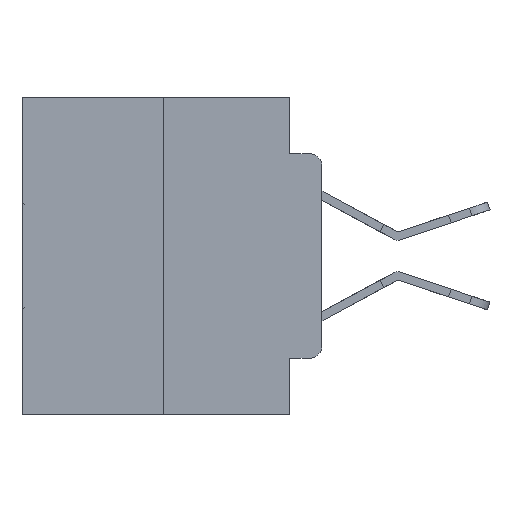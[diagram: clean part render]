
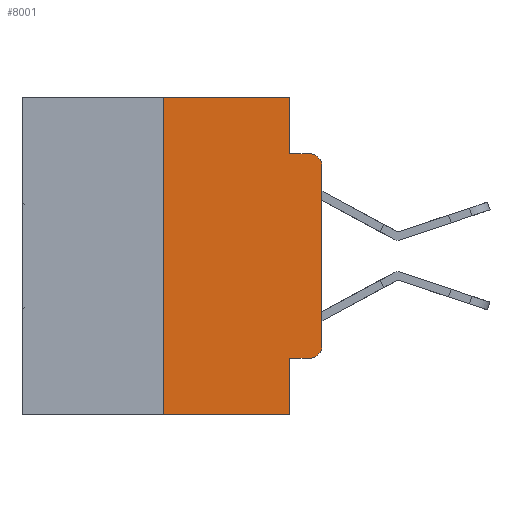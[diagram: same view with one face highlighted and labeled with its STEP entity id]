
A CAD part, left-side view. The second image highlights one B-rep face of the part: STEP entity #8001.
In plain terms, the highlighted planar face has unit normal (-1, 0, 0).
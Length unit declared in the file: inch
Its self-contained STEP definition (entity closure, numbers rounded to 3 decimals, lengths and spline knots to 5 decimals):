
#246 = VERTEX_POINT ( 'NONE', #6823 ) ;
#433 = EDGE_CURVE ( 'NONE', #11601, #15321, #3343, .T. ) ;
#1940 = CARTESIAN_POINT ( 'NONE',  ( 0., 0.02, -0.4115 ) ) ;
#2152 = LINE ( 'NONE', #27426, #26834 ) ;
#2214 = ORIENTED_EDGE ( 'NONE', *, *, #11954, .T. ) ;
#2532 = ORIENTED_EDGE ( 'NONE', *, *, #14152, .F. ) ;
#3255 = EDGE_CURVE ( 'NONE', #19969, #15321, #6133, .T. ) ;
#3343 = LINE ( 'NONE', #30752, #22006 ) ;
#3483 = EDGE_CURVE ( 'NONE', #5431, #4644, #4280, .T. ) ;
#3608 = CARTESIAN_POINT ( 'NONE',  ( 0., 0., -0.3915 ) ) ;
#3788 = CARTESIAN_POINT ( 'NONE',  ( 0., 0.02, -0.0885 ) ) ;
#4202 = EDGE_CURVE ( 'NONE', #11601, #246, #11299, .T. ) ;
#4280 = LINE ( 'NONE', #8751, #16219 ) ;
#4644 = VERTEX_POINT ( 'NONE', #3788 ) ;
#5431 = VERTEX_POINT ( 'NONE', #14275 ) ;
#5774 = PLANE ( 'NONE',  #16772 ) ;
#5930 = DIRECTION ( 'NONE',  ( -1., 0., 0. ) ) ;
#6040 = CARTESIAN_POINT ( 'NONE',  ( 0., 0.02, -0.1085 ) ) ;
#6133 = LINE ( 'NONE', #27066, #17365 ) ;
#6452 = DIRECTION ( 'NONE',  ( -1., 0., 0. ) ) ;
#6823 = CARTESIAN_POINT ( 'NONE',  ( 0., 0.25, 0. ) ) ;
#7395 = CARTESIAN_POINT ( 'NONE',  ( 0., 0.051, 0. ) ) ;
#7549 = VERTEX_POINT ( 'NONE', #16477 ) ;
#7590 = DIRECTION ( 'NONE',  ( 0., 0., -1. ) ) ;
#7930 = ORIENTED_EDGE ( 'NONE', *, *, #27833, .T. ) ;
#8001 = ADVANCED_FACE ( 'NONE', ( #8722 ), #5774, .F. ) ;
#8009 = VERTEX_POINT ( 'NONE', #3608 ) ;
#8514 = ORIENTED_EDGE ( 'NONE', *, *, #3255, .F. ) ;
#8722 = FACE_OUTER_BOUND ( 'NONE', #22912, .T. ) ;
#8751 = CARTESIAN_POINT ( 'NONE',  ( 0., 0.051, -0.0885 ) ) ;
#9223 = ORIENTED_EDGE ( 'NONE', *, *, #3483, .F. ) ;
#9271 = CARTESIAN_POINT ( 'NONE',  ( 0., 0., -0.1085 ) ) ;
#10031 = CARTESIAN_POINT ( 'NONE',  ( 0., 0.051, -0.4115 ) ) ;
#10370 = DIRECTION ( 'NONE',  ( 0., 0., 1. ) ) ;
#10513 = EDGE_CURVE ( 'NONE', #246, #7549, #16839, .T. ) ;
#11299 = LINE ( 'NONE', #25445, #20249 ) ;
#11601 = VERTEX_POINT ( 'NONE', #18677 ) ;
#11954 = EDGE_CURVE ( 'NONE', #19969, #25583, #2152, .T. ) ;
#13089 = DIRECTION ( 'NONE',  ( 1., 0., 0. ) ) ;
#13107 = VECTOR ( 'NONE', #21830, 39.37008 ) ;
#13249 = AXIS2_PLACEMENT_3D ( 'NONE', #6040, #5930, #27075 ) ;
#13459 = DIRECTION ( 'NONE',  ( 0., 0., -1. ) ) ;
#14152 = EDGE_CURVE ( 'NONE', #7549, #5431, #26168, .T. ) ;
#14275 = CARTESIAN_POINT ( 'NONE',  ( 0., 0.051, -0.0885 ) ) ;
#15321 = VERTEX_POINT ( 'NONE', #20814 ) ;
#15499 = DIRECTION ( 'NONE',  ( 0., 0., -1. ) ) ;
#15540 = DIRECTION ( 'NONE',  ( 0., -1., 0. ) ) ;
#15926 = DIRECTION ( 'NONE',  ( 0., 0., 1. ) ) ;
#16219 = VECTOR ( 'NONE', #15540, 39.37008 ) ;
#16477 = CARTESIAN_POINT ( 'NONE',  ( 0., 0.051, 0. ) ) ;
#16772 = AXIS2_PLACEMENT_3D ( 'NONE', #24996, #13089, #15499 ) ;
#16839 = LINE ( 'NONE', #21631, #13107 ) ;
#17365 = VECTOR ( 'NONE', #22522, 39.37008 ) ;
#17809 = VERTEX_POINT ( 'NONE', #9271 ) ;
#18624 = CIRCLE ( 'NONE', #20260, 0.02 ) ;
#18677 = CARTESIAN_POINT ( 'NONE',  ( 0., 0.25, -0.5 ) ) ;
#19781 = VECTOR ( 'NONE', #7590, 39.37008 ) ;
#19969 = VERTEX_POINT ( 'NONE', #10031 ) ;
#19970 = ORIENTED_EDGE ( 'NONE', *, *, #433, .T. ) ;
#20072 = DIRECTION ( 'NONE',  ( 0., -1., 0. ) ) ;
#20249 = VECTOR ( 'NONE', #15926, 39.37008 ) ;
#20260 = AXIS2_PLACEMENT_3D ( 'NONE', #23148, #6452, #13459 ) ;
#20814 = CARTESIAN_POINT ( 'NONE',  ( 0., 0.051, -0.5 ) ) ;
#20967 = LINE ( 'NONE', #27003, #29578 ) ;
#21631 = CARTESIAN_POINT ( 'NONE',  ( 0., 0.473, 0. ) ) ;
#21803 = EDGE_CURVE ( 'NONE', #17809, #4644, #24938, .T. ) ;
#21830 = DIRECTION ( 'NONE',  ( 0., -1., 0. ) ) ;
#22006 = VECTOR ( 'NONE', #22955, 39.37008 ) ;
#22522 = DIRECTION ( 'NONE',  ( 0., 0., -1. ) ) ;
#22912 = EDGE_LOOP ( 'NONE', ( #23474, #26665, #9223, #2532, #28223, #24579, #19970, #8514, #2214, #7930 ) ) ;
#22955 = DIRECTION ( 'NONE',  ( 0., -1., 0. ) ) ;
#23148 = CARTESIAN_POINT ( 'NONE',  ( 0., 0.02, -0.3915 ) ) ;
#23474 = ORIENTED_EDGE ( 'NONE', *, *, #25813, .T. ) ;
#24579 = ORIENTED_EDGE ( 'NONE', *, *, #4202, .F. ) ;
#24938 = CIRCLE ( 'NONE', #13249, 0.02 ) ;
#24996 = CARTESIAN_POINT ( 'NONE',  ( 0., 0.473, 0. ) ) ;
#25445 = CARTESIAN_POINT ( 'NONE',  ( 0., 0.25, 0. ) ) ;
#25583 = VERTEX_POINT ( 'NONE', #1940 ) ;
#25813 = EDGE_CURVE ( 'NONE', #8009, #17809, #20967, .T. ) ;
#26168 = LINE ( 'NONE', #7395, #19781 ) ;
#26665 = ORIENTED_EDGE ( 'NONE', *, *, #21803, .T. ) ;
#26834 = VECTOR ( 'NONE', #20072, 39.37008 ) ;
#27003 = CARTESIAN_POINT ( 'NONE',  ( 0., 0., 0. ) ) ;
#27066 = CARTESIAN_POINT ( 'NONE',  ( 0., 0.051, 0. ) ) ;
#27075 = DIRECTION ( 'NONE',  ( 0., 0., -1. ) ) ;
#27426 = CARTESIAN_POINT ( 'NONE',  ( 0., 0.051, -0.4115 ) ) ;
#27833 = EDGE_CURVE ( 'NONE', #25583, #8009, #18624, .T. ) ;
#28223 = ORIENTED_EDGE ( 'NONE', *, *, #10513, .F. ) ;
#29578 = VECTOR ( 'NONE', #10370, 39.37008 ) ;
#30752 = CARTESIAN_POINT ( 'NONE',  ( 0., 0.473, -0.5 ) ) ;
